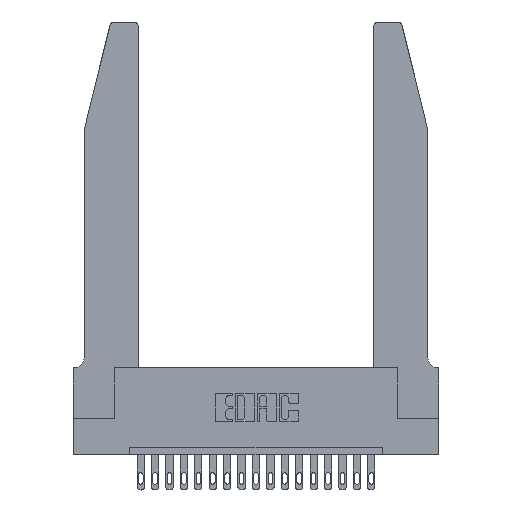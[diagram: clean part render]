
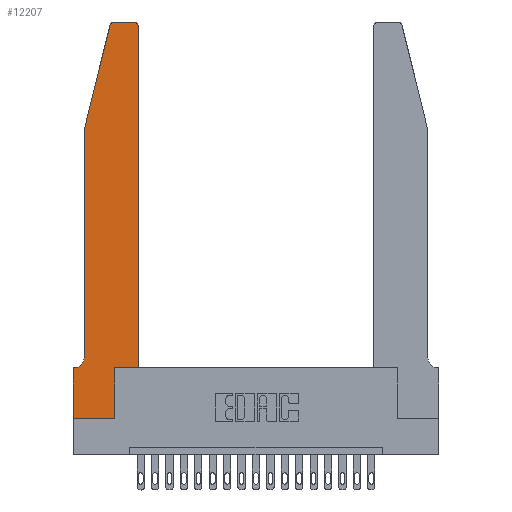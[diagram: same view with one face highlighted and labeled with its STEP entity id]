
A CAD part, top view. The second image highlights one B-rep face of the part: STEP entity #12207.
In plain terms, the highlighted planar face has unit normal (0, 0, 1).
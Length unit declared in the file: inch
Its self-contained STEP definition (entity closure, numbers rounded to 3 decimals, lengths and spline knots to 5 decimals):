
#47 = EDGE_CURVE ( 'NONE', #5946, #1931, #12783, .T. ) ;
#166 = LINE ( 'NONE', #14871, #16778 ) ;
#483 = AXIS2_PLACEMENT_3D ( 'NONE', #15489, #2609, #20207 ) ;
#901 = DIRECTION ( 'NONE',  ( 0., 1., 0. ) ) ;
#1678 = VERTEX_POINT ( 'NONE', #6454 ) ;
#1833 = EDGE_CURVE ( 'NONE', #11368, #10215, #11544, .T. ) ;
#1931 = VERTEX_POINT ( 'NONE', #4749 ) ;
#2193 = CARTESIAN_POINT ( 'NONE',  ( 0.0755, 2., 0.37 ) ) ;
#2324 = DIRECTION ( 'NONE',  ( 0., -1., 0. ) ) ;
#2490 = VECTOR ( 'NONE', #2324, 39.37008 ) ;
#2516 = DIRECTION ( 'NONE',  ( 1., 0., 0. ) ) ;
#2550 = PLANE ( 'NONE',  #483 ) ;
#2609 = DIRECTION ( 'NONE',  ( 0., 0., 1. ) ) ;
#2991 = DIRECTION ( 'NONE',  ( 1., 0., 0. ) ) ;
#3435 = AXIS2_PLACEMENT_3D ( 'NONE', #20364, #12061, #2516 ) ;
#3901 = VECTOR ( 'NONE', #17895, 39.37008 ) ;
#4454 = CARTESIAN_POINT ( 'NONE',  ( 0.0755, 0.35, 0.37 ) ) ;
#4591 = DIRECTION ( 'NONE',  ( 0., 0., -1. ) ) ;
#4749 = CARTESIAN_POINT ( 'NONE',  ( 0., 0., 0.37 ) ) ;
#5112 = EDGE_CURVE ( 'NONE', #5653, #16447, #5466, .T. ) ;
#5466 = CIRCLE ( 'NONE', #8138, 0.07 ) ;
#5569 = DIRECTION ( 'NONE',  ( -1., 0., 0. ) ) ;
#5653 = VERTEX_POINT ( 'NONE', #19483 ) ;
#5818 = ORIENTED_EDGE ( 'NONE', *, *, #18049, .T. ) ;
#5926 = VECTOR ( 'NONE', #5569, 39.37008 ) ;
#5946 = VERTEX_POINT ( 'NONE', #19837 ) ;
#6417 = EDGE_CURVE ( 'NONE', #14531, #1678, #12245, .T. ) ;
#6454 = CARTESIAN_POINT ( 'NONE',  ( 0.4505, 2.72, 0.37 ) ) ;
#6580 = VERTEX_POINT ( 'NONE', #19952 ) ;
#6691 = LINE ( 'NONE', #4454, #5926 ) ;
#6895 = CARTESIAN_POINT ( 'NONE',  ( 0.4505, 0.35, 0.37 ) ) ;
#7007 = DIRECTION ( 'NONE',  ( 0., 0., 1. ) ) ;
#7211 = CARTESIAN_POINT ( 'NONE',  ( 0.2865, 0.35, 0.37 ) ) ;
#7271 = VECTOR ( 'NONE', #9236, 39.37008 ) ;
#7296 = CARTESIAN_POINT ( 'NONE',  ( 0.4505, 0.35, 0.37 ) ) ;
#7677 = VECTOR ( 'NONE', #15450, 39.37008 ) ;
#7743 = CARTESIAN_POINT ( 'NONE',  ( 0.0055, 0.42, 0.37 ) ) ;
#7848 = EDGE_CURVE ( 'NONE', #10215, #14531, #12452, .T. ) ;
#7962 = VECTOR ( 'NONE', #901, 39.37008 ) ;
#8138 = AXIS2_PLACEMENT_3D ( 'NONE', #7743, #4591, #12606 ) ;
#8147 = CARTESIAN_POINT ( 'NONE',  ( 0.4505, 0.35, 0.37 ) ) ;
#8199 = ORIENTED_EDGE ( 'NONE', *, *, #10841, .T. ) ;
#9035 = ORIENTED_EDGE ( 'NONE', *, *, #17261, .T. ) ;
#9236 = DIRECTION ( 'NONE',  ( 0., 1., 0. ) ) ;
#9584 = CARTESIAN_POINT ( 'NONE',  ( 0.284, 2.75, 0.37 ) ) ;
#9684 = CIRCLE ( 'NONE', #3435, 0.03 ) ;
#9770 = ORIENTED_EDGE ( 'NONE', *, *, #7848, .T. ) ;
#9940 = CARTESIAN_POINT ( 'NONE',  ( 0.2865, 0., 0.37 ) ) ;
#10108 = EDGE_CURVE ( 'NONE', #12920, #20178, #166, .T. ) ;
#10215 = VERTEX_POINT ( 'NONE', #18780 ) ;
#10300 = ORIENTED_EDGE ( 'NONE', *, *, #10108, .T. ) ;
#10760 = CARTESIAN_POINT ( 'NONE',  ( 0.0755, 2., 0.37 ) ) ;
#10841 = EDGE_CURVE ( 'NONE', #6580, #5653, #14238, .T. ) ;
#11368 = VERTEX_POINT ( 'NONE', #9940 ) ;
#11544 = LINE ( 'NONE', #7211, #7271 ) ;
#11559 = ORIENTED_EDGE ( 'NONE', *, *, #6417, .T. ) ;
#12061 = DIRECTION ( 'NONE',  ( 0., 0., 1. ) ) ;
#12207 = ADVANCED_FACE ( 'NONE', ( #12916 ), #2550, .T. ) ;
#12245 = LINE ( 'NONE', #7296, #7962 ) ;
#12452 = LINE ( 'NONE', #6895, #3901 ) ;
#12606 = DIRECTION ( 'NONE',  ( -1., 0., 0. ) ) ;
#12783 = LINE ( 'NONE', #16392, #2490 ) ;
#12916 = FACE_OUTER_BOUND ( 'NONE', #16734, .T. ) ;
#12920 = VERTEX_POINT ( 'NONE', #16044 ) ;
#13112 = LINE ( 'NONE', #14305, #19677 ) ;
#13419 = EDGE_CURVE ( 'NONE', #1931, #11368, #13112, .T. ) ;
#13428 = DIRECTION ( 'NONE',  ( -0.239, -0.971, 0. ) ) ;
#14238 = LINE ( 'NONE', #10760, #7677 ) ;
#14305 = CARTESIAN_POINT ( 'NONE',  ( 0., 0., 0.37 ) ) ;
#14331 = ORIENTED_EDGE ( 'NONE', *, *, #17400, .T. ) ;
#14531 = VERTEX_POINT ( 'NONE', #8147 ) ;
#14871 = CARTESIAN_POINT ( 'NONE',  ( 0.2605, 2.75, 0.37 ) ) ;
#15450 = DIRECTION ( 'NONE',  ( 0., -1., 0. ) ) ;
#15489 = CARTESIAN_POINT ( 'NONE',  ( 0., 0.35, 0.37 ) ) ;
#16044 = CARTESIAN_POINT ( 'NONE',  ( 0.4205, 2.75, 0.37 ) ) ;
#16392 = CARTESIAN_POINT ( 'NONE',  ( 0., 0., 0.37 ) ) ;
#16447 = VERTEX_POINT ( 'NONE', #19699 ) ;
#16524 = DIRECTION ( 'NONE',  ( 1., 0., 0. ) ) ;
#16734 = EDGE_LOOP ( 'NONE', ( #10300, #5818, #14331, #8199, #18705, #9035, #17003, #18946, #17603, #9770, #11559, #17959 ) ) ;
#16778 = VECTOR ( 'NONE', #18383, 39.37008 ) ;
#16936 = CARTESIAN_POINT ( 'NONE',  ( 0.25487, 2.72718, 0.37 ) ) ;
#17003 = ORIENTED_EDGE ( 'NONE', *, *, #47, .T. ) ;
#17261 = EDGE_CURVE ( 'NONE', #16447, #5946, #6691, .T. ) ;
#17400 = EDGE_CURVE ( 'NONE', #19861, #6580, #17778, .T. ) ;
#17603 = ORIENTED_EDGE ( 'NONE', *, *, #1833, .T. ) ;
#17700 = CIRCLE ( 'NONE', #19223, 0.03 ) ;
#17778 = LINE ( 'NONE', #2193, #18784 ) ;
#17895 = DIRECTION ( 'NONE',  ( 1., 0., 0. ) ) ;
#17959 = ORIENTED_EDGE ( 'NONE', *, *, #19093, .T. ) ;
#18007 = CARTESIAN_POINT ( 'NONE',  ( 0.4205, 2.72, 0.37 ) ) ;
#18049 = EDGE_CURVE ( 'NONE', #20178, #19861, #9684, .T. ) ;
#18383 = DIRECTION ( 'NONE',  ( -1., 0., 0. ) ) ;
#18705 = ORIENTED_EDGE ( 'NONE', *, *, #5112, .T. ) ;
#18780 = CARTESIAN_POINT ( 'NONE',  ( 0.2865, 0.35, 0.37 ) ) ;
#18784 = VECTOR ( 'NONE', #13428, 39.37008 ) ;
#18946 = ORIENTED_EDGE ( 'NONE', *, *, #13419, .T. ) ;
#19093 = EDGE_CURVE ( 'NONE', #1678, #12920, #17700, .T. ) ;
#19223 = AXIS2_PLACEMENT_3D ( 'NONE', #18007, #7007, #16524 ) ;
#19483 = CARTESIAN_POINT ( 'NONE',  ( 0.0755, 0.42, 0.37 ) ) ;
#19677 = VECTOR ( 'NONE', #2991, 39.37008 ) ;
#19699 = CARTESIAN_POINT ( 'NONE',  ( 0.0055, 0.35, 0.37 ) ) ;
#19837 = CARTESIAN_POINT ( 'NONE',  ( 0., 0.35, 0.37 ) ) ;
#19861 = VERTEX_POINT ( 'NONE', #16936 ) ;
#19952 = CARTESIAN_POINT ( 'NONE',  ( 0.0755, 2., 0.37 ) ) ;
#20178 = VERTEX_POINT ( 'NONE', #9584 ) ;
#20207 = DIRECTION ( 'NONE',  ( 1., 0., 0. ) ) ;
#20364 = CARTESIAN_POINT ( 'NONE',  ( 0.284, 2.72, 0.37 ) ) ;
